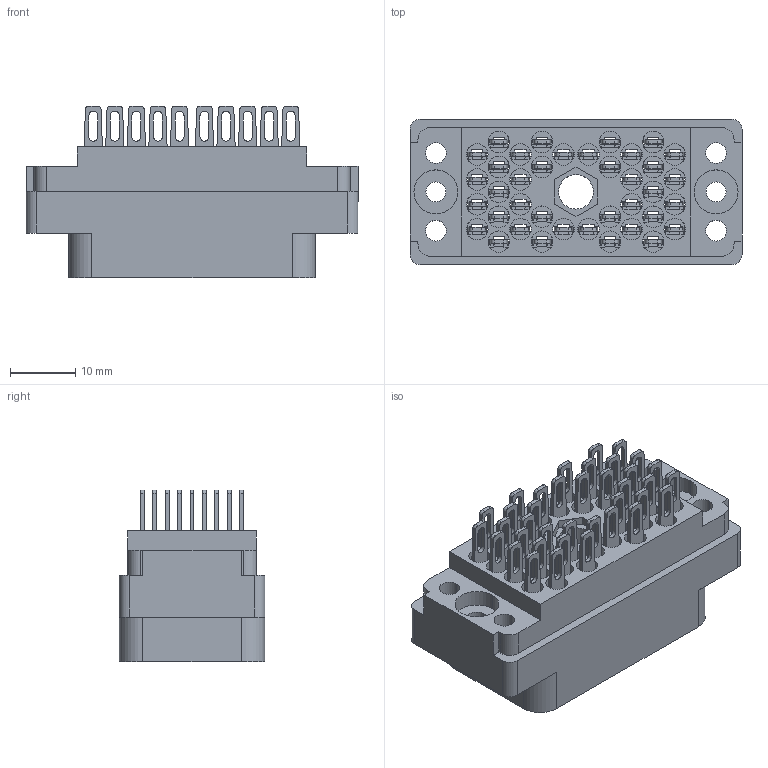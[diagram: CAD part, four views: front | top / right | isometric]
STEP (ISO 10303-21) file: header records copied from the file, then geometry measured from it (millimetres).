
FILE_DESCRIPTION (( 'STEP AP203' ), '1' );
FILE_NAME ('516-038-500-300.STEP', '2020-03-09T19:42:35', ( '' ), ( '' ), 'SwSTEP 2.0', 'SolidWorks 2016', '' );
FILE_SCHEMA (( 'CONFIG_CONTROL_DESIGN' ));
Length unit declared in the file: inch
Products named in the file (3): 516-292-001_500 Contact; 516 Plug Insulator_038; 516-038-500-300
Assembly tree (39 placements, depth 2):
  516-038-500-300
    516 Plug Insulator_038
    516-292-001_500 Contact  x38
Bounding box: 50.8 x 22.25 x 26.26 mm (x, y, z)
Volume: 10045.6 mm3; surface area: 18358.1 mm2
Topology: 39 solids, 39 shells, 3774 faces, 10960 edges, 7280 vertices
Faces by surface type: plane 2275, cylinder 1269, bspline 228, cone 2
Entity records: 33794 total; most frequent: CARTESIAN_POINT 5987, ORIENTED_EDGE 5640, DIRECTION 5466, EDGE_CURVE 2820, VECTOR 2102, LINE 2102, VERTEX_POINT 1878, AXIS2_PLACEMENT_3D 1682
